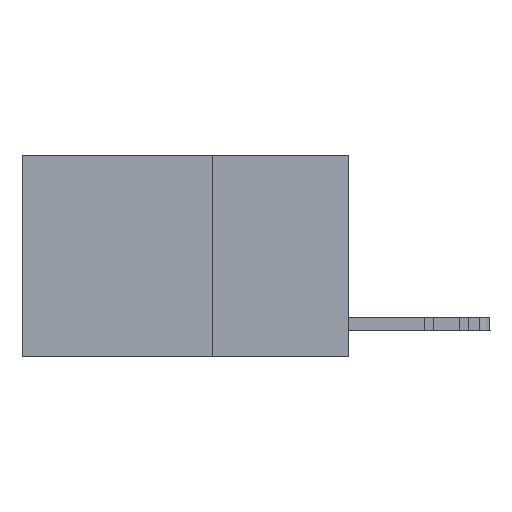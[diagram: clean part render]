
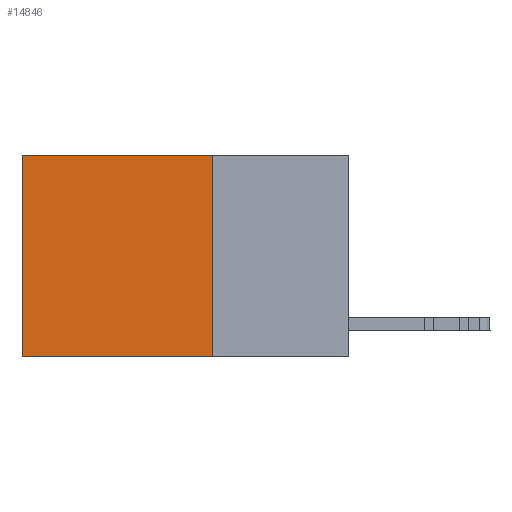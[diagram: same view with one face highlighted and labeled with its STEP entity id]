
A CAD part, left-side view. The second image highlights one B-rep face of the part: STEP entity #14846.
In plain terms, the highlighted planar face has unit normal (-1, 0, 0).
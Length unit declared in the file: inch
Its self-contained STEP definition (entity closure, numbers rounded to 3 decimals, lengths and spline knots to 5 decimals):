
#259 = ORIENTED_EDGE ( 'NONE', *, *, #22720, .T. ) ;
#1026 = VERTEX_POINT ( 'NONE', #7573 ) ;
#2289 = ORIENTED_EDGE ( 'NONE', *, *, #7100, .T. ) ;
#2782 = VECTOR ( 'NONE', #26781, 39.37008 ) ;
#3578 = CARTESIAN_POINT ( 'NONE',  ( 0.2625, 0.25, 0. ) ) ;
#4254 = EDGE_CURVE ( 'NONE', #14950, #23746, #26176, .T. ) ;
#6186 = VERTEX_POINT ( 'NONE', #26582 ) ;
#6853 = LINE ( 'NONE', #15872, #23067 ) ;
#7100 = EDGE_CURVE ( 'NONE', #1026, #6186, #6853, .T. ) ;
#7163 = EDGE_CURVE ( 'NONE', #23746, #6186, #11132, .T. ) ;
#7573 = CARTESIAN_POINT ( 'NONE',  ( 0.2625, 0.6, 0. ) ) ;
#7580 = PLANE ( 'NONE',  #8138 ) ;
#8138 = AXIS2_PLACEMENT_3D ( 'NONE', #23537, #12155, #28106 ) ;
#9065 = VECTOR ( 'NONE', #13009, 39.37008 ) ;
#9467 = CARTESIAN_POINT ( 'NONE',  ( 0.2625, 0.25, 0. ) ) ;
#11132 = LINE ( 'NONE', #11420, #2782 ) ;
#11420 = CARTESIAN_POINT ( 'NONE',  ( 0.2625, 0.25, -0.37 ) ) ;
#12155 = DIRECTION ( 'NONE',  ( 1., 0., 0. ) ) ;
#12187 = VECTOR ( 'NONE', #27065, 39.37008 ) ;
#12728 = CARTESIAN_POINT ( 'NONE',  ( 0.2625, 0.25, -0.37 ) ) ;
#13009 = DIRECTION ( 'NONE',  ( 0., 0., -1. ) ) ;
#14846 = ADVANCED_FACE ( 'NONE', ( #18825 ), #7580, .F. ) ;
#14950 = VERTEX_POINT ( 'NONE', #28826 ) ;
#15858 = LINE ( 'NONE', #9467, #12187 ) ;
#15872 = CARTESIAN_POINT ( 'NONE',  ( 0.2625, 0.6, 0. ) ) ;
#18825 = FACE_OUTER_BOUND ( 'NONE', #20127, .T. ) ;
#20127 = EDGE_LOOP ( 'NONE', ( #2289, #23210, #25965, #259 ) ) ;
#22720 = EDGE_CURVE ( 'NONE', #14950, #1026, #15858, .T. ) ;
#23067 = VECTOR ( 'NONE', #24876, 39.37008 ) ;
#23210 = ORIENTED_EDGE ( 'NONE', *, *, #7163, .F. ) ;
#23537 = CARTESIAN_POINT ( 'NONE',  ( 0.2625, 0.25, 0. ) ) ;
#23746 = VERTEX_POINT ( 'NONE', #12728 ) ;
#24876 = DIRECTION ( 'NONE',  ( 0., 0., -1. ) ) ;
#25965 = ORIENTED_EDGE ( 'NONE', *, *, #4254, .F. ) ;
#26176 = LINE ( 'NONE', #3578, #9065 ) ;
#26582 = CARTESIAN_POINT ( 'NONE',  ( 0.2625, 0.6, -0.37 ) ) ;
#26781 = DIRECTION ( 'NONE',  ( 0., 1., 0. ) ) ;
#27065 = DIRECTION ( 'NONE',  ( 0., 1., 0. ) ) ;
#28106 = DIRECTION ( 'NONE',  ( 0., 0., -1. ) ) ;
#28826 = CARTESIAN_POINT ( 'NONE',  ( 0.2625, 0.25, 0. ) ) ;
